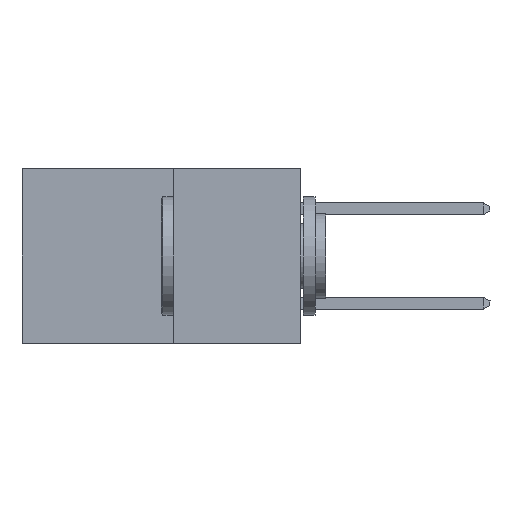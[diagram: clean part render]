
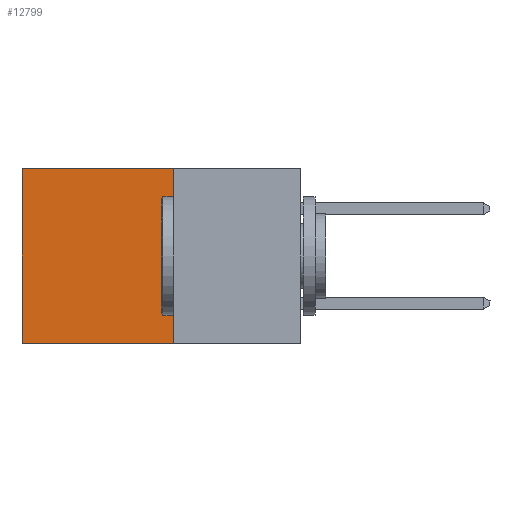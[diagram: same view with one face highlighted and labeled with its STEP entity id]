
A CAD part, left-side view. The second image highlights one B-rep face of the part: STEP entity #12799.
In plain terms, the highlighted planar face has unit normal (-1, 0, 0).
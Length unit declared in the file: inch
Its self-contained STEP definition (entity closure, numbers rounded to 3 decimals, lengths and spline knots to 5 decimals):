
#376 = VECTOR ( 'NONE', #1353, 39.37008 ) ;
#591 = CARTESIAN_POINT ( 'NONE',  ( 0.277, 0.59, -0.37 ) ) ;
#721 = LINE ( 'NONE', #4466, #376 ) ;
#1114 = ORIENTED_EDGE ( 'NONE', *, *, #7131, .T. ) ;
#1353 = DIRECTION ( 'NONE',  ( 0., 1., 0. ) ) ;
#1477 = CARTESIAN_POINT ( 'NONE',  ( 0.277, 0.27, 0. ) ) ;
#1496 = ORIENTED_EDGE ( 'NONE', *, *, #12055, .F. ) ;
#2003 = EDGE_CURVE ( 'NONE', #2384, #10945, #10917, .T. ) ;
#2096 = EDGE_CURVE ( 'NONE', #2384, #8317, #12891, .T. ) ;
#2384 = VERTEX_POINT ( 'NONE', #1477 ) ;
#3088 = LINE ( 'NONE', #6269, #3413 ) ;
#3142 = AXIS2_PLACEMENT_3D ( 'NONE', #7725, #9741, #3621 ) ;
#3413 = VECTOR ( 'NONE', #6021, 39.37008 ) ;
#3621 = DIRECTION ( 'NONE',  ( 0., 0., -1. ) ) ;
#3871 = CARTESIAN_POINT ( 'NONE',  ( 0.277, 0.27, -0.37 ) ) ;
#4039 = CARTESIAN_POINT ( 'NONE',  ( 0.277, 0.59, 0. ) ) ;
#4466 = CARTESIAN_POINT ( 'NONE',  ( 0.277, 0.27, -0.37 ) ) ;
#4838 = CARTESIAN_POINT ( 'NONE',  ( 0.277, 0.27, 0. ) ) ;
#5266 = CARTESIAN_POINT ( 'NONE',  ( 0.277, 0.27, -0.37 ) ) ;
#5521 = VECTOR ( 'NONE', #11302, 39.37008 ) ;
#6021 = DIRECTION ( 'NONE',  ( 0., 0., -1. ) ) ;
#6269 = CARTESIAN_POINT ( 'NONE',  ( 0.277, 0.59, -0.37 ) ) ;
#7131 = EDGE_CURVE ( 'NONE', #10945, #12228, #3088, .T. ) ;
#7549 = FACE_OUTER_BOUND ( 'NONE', #7731, .T. ) ;
#7725 = CARTESIAN_POINT ( 'NONE',  ( 0.277, 0.27, -0.37 ) ) ;
#7731 = EDGE_LOOP ( 'NONE', ( #1114, #1496, #8094, #13113 ) ) ;
#8094 = ORIENTED_EDGE ( 'NONE', *, *, #2096, .F. ) ;
#8317 = VERTEX_POINT ( 'NONE', #3871 ) ;
#8721 = PLANE ( 'NONE',  #3142 ) ;
#9637 = DIRECTION ( 'NONE',  ( 0., 0., -1. ) ) ;
#9741 = DIRECTION ( 'NONE',  ( 1., 0., 0. ) ) ;
#10917 = LINE ( 'NONE', #4838, #5521 ) ;
#10945 = VERTEX_POINT ( 'NONE', #4039 ) ;
#11302 = DIRECTION ( 'NONE',  ( 0., 1., 0. ) ) ;
#12055 = EDGE_CURVE ( 'NONE', #8317, #12228, #721, .T. ) ;
#12228 = VERTEX_POINT ( 'NONE', #591 ) ;
#12296 = VECTOR ( 'NONE', #9637, 39.37008 ) ;
#12799 = ADVANCED_FACE ( 'NONE', ( #7549 ), #8721, .F. ) ;
#12891 = LINE ( 'NONE', #5266, #12296 ) ;
#13113 = ORIENTED_EDGE ( 'NONE', *, *, #2003, .T. ) ;
